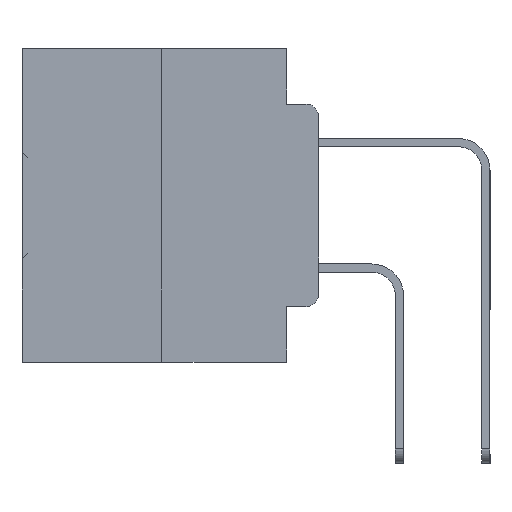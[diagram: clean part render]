
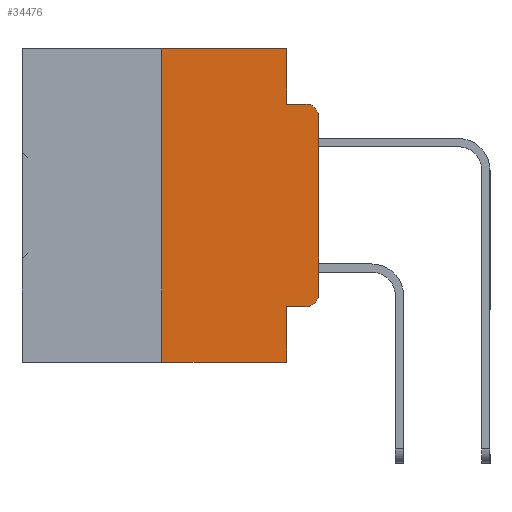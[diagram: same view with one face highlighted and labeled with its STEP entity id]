
A CAD part, left-side view. The second image highlights one B-rep face of the part: STEP entity #34476.
In plain terms, the highlighted planar face has unit normal (-1, 0, 0).
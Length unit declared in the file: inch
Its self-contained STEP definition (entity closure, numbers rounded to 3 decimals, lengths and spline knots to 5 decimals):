
#914 = ORIENTED_EDGE ( 'NONE', *, *, #25213, .T. ) ;
#954 = EDGE_CURVE ( 'NONE', #27147, #25621, #34527, .T. ) ;
#1609 = VECTOR ( 'NONE', #22359, 39.37008 ) ;
#2004 = CARTESIAN_POINT ( 'NONE',  ( 0., 0.051, 0. ) ) ;
#2079 = CARTESIAN_POINT ( 'NONE',  ( 0., 0.02, -0.3915 ) ) ;
#2967 = EDGE_CURVE ( 'NONE', #25621, #14007, #32912, .T. ) ;
#3237 = CARTESIAN_POINT ( 'NONE',  ( 0., 0.02, -0.1085 ) ) ;
#4822 = VERTEX_POINT ( 'NONE', #29396 ) ;
#4886 = EDGE_CURVE ( 'NONE', #14932, #14007, #13375, .T. ) ;
#4985 = DIRECTION ( 'NONE',  ( 0., 0., -1. ) ) ;
#5033 = ORIENTED_EDGE ( 'NONE', *, *, #35205, .F. ) ;
#5321 = CARTESIAN_POINT ( 'NONE',  ( 0., 0.473, 0. ) ) ;
#6147 = DIRECTION ( 'NONE',  ( 0., 0., -1. ) ) ;
#6908 = DIRECTION ( 'NONE',  ( 1., 0., 0. ) ) ;
#7370 = VERTEX_POINT ( 'NONE', #22125 ) ;
#7644 = FACE_OUTER_BOUND ( 'NONE', #30234, .T. ) ;
#8746 = VECTOR ( 'NONE', #16451, 39.37008 ) ;
#9217 = ORIENTED_EDGE ( 'NONE', *, *, #29365, .T. ) ;
#9624 = ORIENTED_EDGE ( 'NONE', *, *, #2967, .F. ) ;
#10450 = CARTESIAN_POINT ( 'NONE',  ( 0., 0.473, -0.5 ) ) ;
#10573 = ORIENTED_EDGE ( 'NONE', *, *, #33262, .F. ) ;
#12389 = CARTESIAN_POINT ( 'NONE',  ( 0., 0.25, -0.5 ) ) ;
#12458 = DIRECTION ( 'NONE',  ( 0., 0., 1. ) ) ;
#12468 = VERTEX_POINT ( 'NONE', #37559 ) ;
#12671 = VECTOR ( 'NONE', #13175, 39.37008 ) ;
#12751 = EDGE_CURVE ( 'NONE', #12468, #14932, #22335, .T. ) ;
#13175 = DIRECTION ( 'NONE',  ( 0., 0., 1. ) ) ;
#13243 = VERTEX_POINT ( 'NONE', #23933 ) ;
#13372 = AXIS2_PLACEMENT_3D ( 'NONE', #15700, #6908, #27591 ) ;
#13375 = CIRCLE ( 'NONE', #33463, 0.02 ) ;
#13404 = DIRECTION ( 'NONE',  ( 0., -1., 0. ) ) ;
#13705 = DIRECTION ( 'NONE',  ( 0., -1., 0. ) ) ;
#14007 = VERTEX_POINT ( 'NONE', #27217 ) ;
#14932 = VERTEX_POINT ( 'NONE', #37714 ) ;
#15196 = CARTESIAN_POINT ( 'NONE',  ( 0., 0.051, -0.0885 ) ) ;
#15668 = ORIENTED_EDGE ( 'NONE', *, *, #12751, .T. ) ;
#15700 = CARTESIAN_POINT ( 'NONE',  ( 0., 0.473, 0. ) ) ;
#16115 = ORIENTED_EDGE ( 'NONE', *, *, #954, .F. ) ;
#16318 = EDGE_CURVE ( 'NONE', #4822, #27147, #26739, .T. ) ;
#16451 = DIRECTION ( 'NONE',  ( 0., 0., -1. ) ) ;
#16577 = AXIS2_PLACEMENT_3D ( 'NONE', #2079, #22700, #4985 ) ;
#16612 = LINE ( 'NONE', #34040, #8746 ) ;
#17946 = VECTOR ( 'NONE', #23038, 39.37008 ) ;
#21427 = CARTESIAN_POINT ( 'NONE',  ( 0., 0.051, -0.4115 ) ) ;
#22125 = CARTESIAN_POINT ( 'NONE',  ( 0., 0.02, -0.4115 ) ) ;
#22273 = VECTOR ( 'NONE', #13404, 39.37008 ) ;
#22316 = VECTOR ( 'NONE', #13705, 39.37008 ) ;
#22335 = LINE ( 'NONE', #30177, #37862 ) ;
#22359 = DIRECTION ( 'NONE',  ( 0., -1., 0. ) ) ;
#22700 = DIRECTION ( 'NONE',  ( -1., 0., 0. ) ) ;
#23038 = DIRECTION ( 'NONE',  ( 0., -1., 0. ) ) ;
#23867 = DIRECTION ( 'NONE',  ( -1., 0., 0. ) ) ;
#23933 = CARTESIAN_POINT ( 'NONE',  ( 0., 0.051, -0.5 ) ) ;
#24629 = PLANE ( 'NONE',  #13372 ) ;
#24934 = VECTOR ( 'NONE', #25765, 39.37008 ) ;
#25213 = EDGE_CURVE ( 'NONE', #33067, #13243, #36877, .T. ) ;
#25398 = ORIENTED_EDGE ( 'NONE', *, *, #4886, .T. ) ;
#25494 = CARTESIAN_POINT ( 'NONE',  ( 0., 0.051, -0.4115 ) ) ;
#25621 = VERTEX_POINT ( 'NONE', #15196 ) ;
#25765 = DIRECTION ( 'NONE',  ( 0., 0., -1. ) ) ;
#25800 = CARTESIAN_POINT ( 'NONE',  ( 0., 0.051, 0. ) ) ;
#26739 = LINE ( 'NONE', #5321, #17946 ) ;
#27147 = VERTEX_POINT ( 'NONE', #2004 ) ;
#27217 = CARTESIAN_POINT ( 'NONE',  ( 0., 0.02, -0.0885 ) ) ;
#27591 = DIRECTION ( 'NONE',  ( 0., 0., -1. ) ) ;
#27807 = CARTESIAN_POINT ( 'NONE',  ( 0., 0.25, 0. ) ) ;
#27935 = LINE ( 'NONE', #27807, #12671 ) ;
#29365 = EDGE_CURVE ( 'NONE', #7370, #12468, #37548, .T. ) ;
#29396 = CARTESIAN_POINT ( 'NONE',  ( 0., 0.25, 0. ) ) ;
#29980 = ORIENTED_EDGE ( 'NONE', *, *, #31315, .T. ) ;
#30177 = CARTESIAN_POINT ( 'NONE',  ( 0., 0., 0. ) ) ;
#30234 = EDGE_LOOP ( 'NONE', ( #15668, #25398, #9624, #16115, #32697, #5033, #914, #10573, #29980, #9217 ) ) ;
#31035 = LINE ( 'NONE', #25494, #22316 ) ;
#31315 = EDGE_CURVE ( 'NONE', #33870, #7370, #31035, .T. ) ;
#32697 = ORIENTED_EDGE ( 'NONE', *, *, #16318, .F. ) ;
#32912 = LINE ( 'NONE', #36892, #1609 ) ;
#33067 = VERTEX_POINT ( 'NONE', #12389 ) ;
#33262 = EDGE_CURVE ( 'NONE', #33870, #13243, #16612, .T. ) ;
#33463 = AXIS2_PLACEMENT_3D ( 'NONE', #3237, #23867, #6147 ) ;
#33870 = VERTEX_POINT ( 'NONE', #21427 ) ;
#34040 = CARTESIAN_POINT ( 'NONE',  ( 0., 0.051, 0. ) ) ;
#34476 = ADVANCED_FACE ( 'NONE', ( #7644 ), #24629, .F. ) ;
#34527 = LINE ( 'NONE', #25800, #24934 ) ;
#35205 = EDGE_CURVE ( 'NONE', #33067, #4822, #27935, .T. ) ;
#36877 = LINE ( 'NONE', #10450, #22273 ) ;
#36892 = CARTESIAN_POINT ( 'NONE',  ( 0., 0.051, -0.0885 ) ) ;
#37548 = CIRCLE ( 'NONE', #16577, 0.02 ) ;
#37559 = CARTESIAN_POINT ( 'NONE',  ( 0., 0., -0.3915 ) ) ;
#37714 = CARTESIAN_POINT ( 'NONE',  ( 0., 0., -0.1085 ) ) ;
#37862 = VECTOR ( 'NONE', #12458, 39.37008 ) ;
